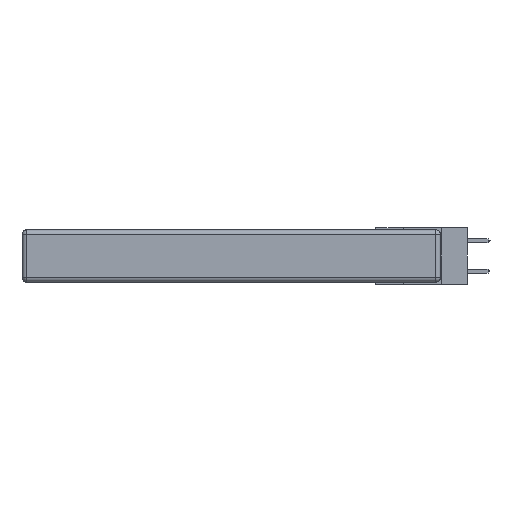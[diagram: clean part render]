
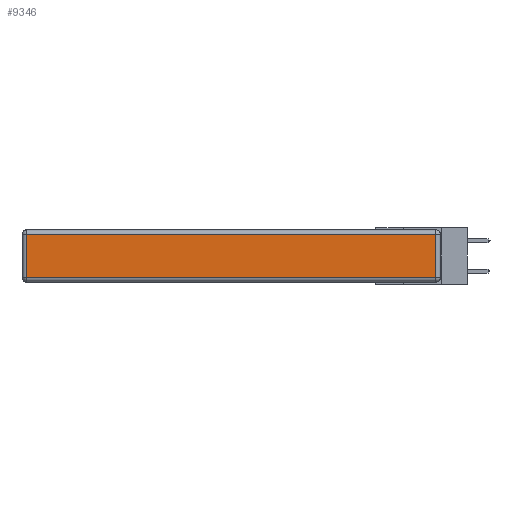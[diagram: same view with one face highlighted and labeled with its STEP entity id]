
A CAD part, left-side view. The second image highlights one B-rep face of the part: STEP entity #9346.
In plain terms, the highlighted planar face has unit normal (-1, 0, 0).
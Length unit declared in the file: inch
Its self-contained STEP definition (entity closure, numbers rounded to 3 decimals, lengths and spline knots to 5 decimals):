
#816 = ORIENTED_EDGE ( 'NONE', *, *, #12956, .T. ) ;
#1592 = DIRECTION ( 'NONE',  ( 0., 0., 1. ) ) ;
#2399 = VERTEX_POINT ( 'NONE', #4695 ) ;
#4060 = PLANE ( 'NONE',  #8109 ) ;
#4695 = CARTESIAN_POINT ( 'NONE',  ( 0., 0.03, -0.313 ) ) ;
#5395 = LINE ( 'NONE', #21123, #7378 ) ;
#5442 = FACE_OUTER_BOUND ( 'NONE', #17161, .T. ) ;
#7378 = VECTOR ( 'NONE', #25258, 39.37008 ) ;
#7981 = VERTEX_POINT ( 'NONE', #19078 ) ;
#8109 = AXIS2_PLACEMENT_3D ( 'NONE', #27324, #27601, #1592 ) ;
#8836 = CARTESIAN_POINT ( 'NONE',  ( 0., 2.72, -0.313 ) ) ;
#9346 = ADVANCED_FACE ( 'NONE', ( #5442 ), #4060, .T. ) ;
#10288 = EDGE_CURVE ( 'NONE', #7981, #14303, #5395, .T. ) ;
#10709 = DIRECTION ( 'NONE',  ( 0., 1., 0. ) ) ;
#11425 = CARTESIAN_POINT ( 'NONE',  ( 0., 0.03, -0.03 ) ) ;
#11607 = LINE ( 'NONE', #23406, #17678 ) ;
#12879 = EDGE_CURVE ( 'NONE', #14303, #2399, #11607, .T. ) ;
#12956 = EDGE_CURVE ( 'NONE', #15255, #7981, #19346, .T. ) ;
#14303 = VERTEX_POINT ( 'NONE', #8836 ) ;
#15016 = VECTOR ( 'NONE', #21411, 39.37008 ) ;
#15255 = VERTEX_POINT ( 'NONE', #11425 ) ;
#15281 = ORIENTED_EDGE ( 'NONE', *, *, #12879, .T. ) ;
#17161 = EDGE_LOOP ( 'NONE', ( #15281, #23455, #816, #17412 ) ) ;
#17412 = ORIENTED_EDGE ( 'NONE', *, *, #10288, .T. ) ;
#17678 = VECTOR ( 'NONE', #27606, 39.37008 ) ;
#18992 = CARTESIAN_POINT ( 'NONE',  ( 0., 2.75, -0.03 ) ) ;
#19078 = CARTESIAN_POINT ( 'NONE',  ( 0., 2.72, -0.03 ) ) ;
#19346 = LINE ( 'NONE', #18992, #20015 ) ;
#20015 = VECTOR ( 'NONE', #10709, 39.37008 ) ;
#21123 = CARTESIAN_POINT ( 'NONE',  ( 0., 2.72, -0.343 ) ) ;
#21411 = DIRECTION ( 'NONE',  ( 0., 0., 1. ) ) ;
#22993 = EDGE_CURVE ( 'NONE', #2399, #15255, #27402, .T. ) ;
#23406 = CARTESIAN_POINT ( 'NONE',  ( 0., 0., -0.313 ) ) ;
#23455 = ORIENTED_EDGE ( 'NONE', *, *, #22993, .T. ) ;
#23672 = CARTESIAN_POINT ( 'NONE',  ( 0., 0.03, -0.343 ) ) ;
#25258 = DIRECTION ( 'NONE',  ( 0., 0., -1. ) ) ;
#27324 = CARTESIAN_POINT ( 'NONE',  ( 0., 0., -0.343 ) ) ;
#27402 = LINE ( 'NONE', #23672, #15016 ) ;
#27601 = DIRECTION ( 'NONE',  ( -1., 0., 0. ) ) ;
#27606 = DIRECTION ( 'NONE',  ( 0., -1., 0. ) ) ;
